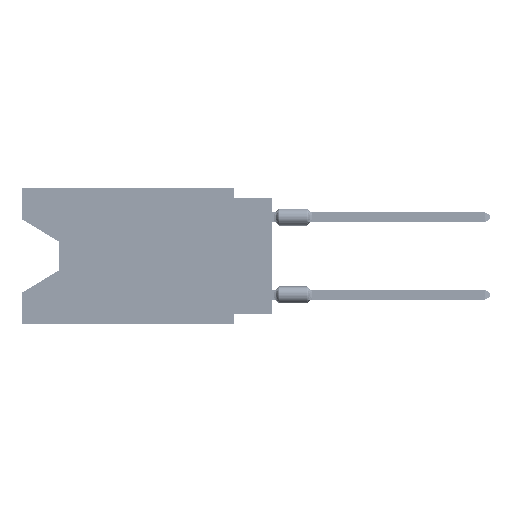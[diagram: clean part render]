
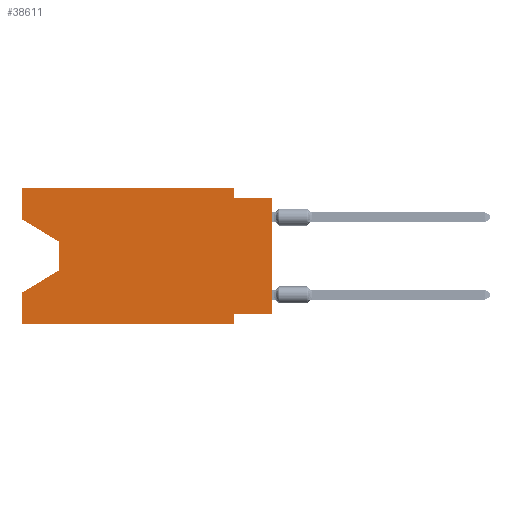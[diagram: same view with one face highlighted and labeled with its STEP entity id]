
A CAD part, left-side view. The second image highlights one B-rep face of the part: STEP entity #38611.
In plain terms, the highlighted planar face has unit normal (-1, 0, 0).
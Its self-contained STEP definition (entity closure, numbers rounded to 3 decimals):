
#2183 = CARTESIAN_POINT ( 'NONE',  ( 0., 2.54, -0.635 ) ) ;
#4354 = EDGE_CURVE ( 'NONE', #25332, #64421, #41586, .T. ) ;
#4647 = EDGE_LOOP ( 'NONE', ( #14590, #85293, #22758, #9300, #32544, #81004, #24702, #36035, #92510, #18713, #27434, #96719 ) ) ;
#5508 = VECTOR ( 'NONE', #71058, 1000. ) ;
#8305 = DIRECTION ( 'NONE',  ( 0., 0., 1. ) ) ;
#8428 = VECTOR ( 'NONE', #8305, 1000. ) ;
#9300 = ORIENTED_EDGE ( 'NONE', *, *, #54876, .F. ) ;
#11261 = EDGE_CURVE ( 'NONE', #54939, #77517, #31250, .T. ) ;
#13982 = CARTESIAN_POINT ( 'NONE',  ( 0., 16.383, -8.89 ) ) ;
#14084 = CARTESIAN_POINT ( 'NONE',  ( 0., 16.383, 0. ) ) ;
#14590 = ORIENTED_EDGE ( 'NONE', *, *, #80963, .T. ) ;
#15507 = LINE ( 'NONE', #75867, #44547 ) ;
#16127 = VECTOR ( 'NONE', #97850, 1000. ) ;
#16807 = VECTOR ( 'NONE', #97459, 1000. ) ;
#16963 = PLANE ( 'NONE',  #18450 ) ;
#18450 = AXIS2_PLACEMENT_3D ( 'NONE', #32440, #55867, #62850 ) ;
#18713 = ORIENTED_EDGE ( 'NONE', *, *, #30971, .F. ) ;
#20438 = CARTESIAN_POINT ( 'NONE',  ( 0., 2.54, 0. ) ) ;
#21786 = EDGE_CURVE ( 'NONE', #24585, #88785, #82406, .T. ) ;
#22758 = ORIENTED_EDGE ( 'NONE', *, *, #77411, .T. ) ;
#24585 = VERTEX_POINT ( 'NONE', #67412 ) ;
#24702 = ORIENTED_EDGE ( 'NONE', *, *, #63121, .F. ) ;
#25153 = CARTESIAN_POINT ( 'NONE',  ( 0., 16.383, -8.89 ) ) ;
#25172 = DIRECTION ( 'NONE',  ( 0., 1., 0. ) ) ;
#25332 = VERTEX_POINT ( 'NONE', #95007 ) ;
#26108 = CARTESIAN_POINT ( 'NONE',  ( 0., 13.97, -3.505 ) ) ;
#27434 = ORIENTED_EDGE ( 'NONE', *, *, #94796, .F. ) ;
#28334 = VECTOR ( 'NONE', #46251, 1000. ) ;
#30971 = EDGE_CURVE ( 'NONE', #33474, #76440, #81770, .T. ) ;
#31250 = LINE ( 'NONE', #76622, #8428 ) ;
#32107 = DIRECTION ( 'NONE',  ( 0., -1., 0. ) ) ;
#32440 = CARTESIAN_POINT ( 'NONE',  ( 0., 16.383, 0. ) ) ;
#32544 = ORIENTED_EDGE ( 'NONE', *, *, #86923, .T. ) ;
#33474 = VERTEX_POINT ( 'NONE', #43548 ) ;
#34459 = VERTEX_POINT ( 'NONE', #25153 ) ;
#35404 = CARTESIAN_POINT ( 'NONE',  ( 0., 16.383, -2.038 ) ) ;
#36035 = ORIENTED_EDGE ( 'NONE', *, *, #11261, .T. ) ;
#36974 = EDGE_CURVE ( 'NONE', #76440, #77517, #76984, .T. ) ;
#37620 = LINE ( 'NONE', #89989, #16807 ) ;
#37853 = VECTOR ( 'NONE', #43571, 1000. ) ;
#38611 = ADVANCED_FACE ( 'NONE', ( #63337 ), #16963, .F. ) ;
#40628 = LINE ( 'NONE', #78994, #85141 ) ;
#41586 = LINE ( 'NONE', #26108, #28334 ) ;
#43147 = VECTOR ( 'NONE', #88784, 1000. ) ;
#43548 = CARTESIAN_POINT ( 'NONE',  ( 0., 2.54, 0. ) ) ;
#43571 = DIRECTION ( 'NONE',  ( 0., 0., 1. ) ) ;
#43998 = DIRECTION ( 'NONE',  ( 0., -1., 0. ) ) ;
#44547 = VECTOR ( 'NONE', #43998, 1000. ) ;
#46251 = DIRECTION ( 'NONE',  ( 0., 0., -1. ) ) ;
#51066 = CARTESIAN_POINT ( 'NONE',  ( 0., 13.97, -5.385 ) ) ;
#52609 = CARTESIAN_POINT ( 'NONE',  ( 0., 0., -0.635 ) ) ;
#54491 = CARTESIAN_POINT ( 'NONE',  ( 0., 16.383, -6.852 ) ) ;
#54876 = EDGE_CURVE ( 'NONE', #34459, #63399, #90419, .T. ) ;
#54939 = VERTEX_POINT ( 'NONE', #93355 ) ;
#55867 = DIRECTION ( 'NONE',  ( 1., 0., 0. ) ) ;
#62258 = VECTOR ( 'NONE', #73878, 1000. ) ;
#62850 = DIRECTION ( 'NONE',  ( 0., 0., -1. ) ) ;
#63121 = EDGE_CURVE ( 'NONE', #54939, #24585, #40628, .T. ) ;
#63337 = FACE_OUTER_BOUND ( 'NONE', #4647, .T. ) ;
#63399 = VERTEX_POINT ( 'NONE', #54491 ) ;
#64421 = VERTEX_POINT ( 'NONE', #51066 ) ;
#65108 = DIRECTION ( 'NONE',  ( 0., 0.855, -0.519 ) ) ;
#65611 = CARTESIAN_POINT ( 'NONE',  ( 0., 13.97, -5.385 ) ) ;
#66101 = LINE ( 'NONE', #65611, #96582 ) ;
#67412 = CARTESIAN_POINT ( 'NONE',  ( 0., 2.54, -8.255 ) ) ;
#68366 = VERTEX_POINT ( 'NONE', #93583 ) ;
#69507 = CARTESIAN_POINT ( 'NONE',  ( 0., 0., -0.635 ) ) ;
#71058 = DIRECTION ( 'NONE',  ( 0., 0., 1. ) ) ;
#73878 = DIRECTION ( 'NONE',  ( 0., -1., 0. ) ) ;
#74101 = CARTESIAN_POINT ( 'NONE',  ( 0., 2.54, -8.89 ) ) ;
#75867 = CARTESIAN_POINT ( 'NONE',  ( 0., 16.383, 0. ) ) ;
#75901 = CARTESIAN_POINT ( 'NONE',  ( 0., 2.54, -8.89 ) ) ;
#76440 = VERTEX_POINT ( 'NONE', #2183 ) ;
#76622 = CARTESIAN_POINT ( 'NONE',  ( 0., 0., 0. ) ) ;
#76984 = LINE ( 'NONE', #69507, #98123 ) ;
#77411 = EDGE_CURVE ( 'NONE', #64421, #63399, #66101, .T. ) ;
#77517 = VERTEX_POINT ( 'NONE', #52609 ) ;
#78539 = CARTESIAN_POINT ( 'NONE',  ( 0., 16.383, 0. ) ) ;
#78994 = CARTESIAN_POINT ( 'NONE',  ( 0., 0., -8.255 ) ) ;
#80963 = EDGE_CURVE ( 'NONE', #83447, #25332, #37620, .T. ) ;
#81004 = ORIENTED_EDGE ( 'NONE', *, *, #21786, .F. ) ;
#81770 = LINE ( 'NONE', #20438, #43147 ) ;
#82406 = LINE ( 'NONE', #75901, #16127 ) ;
#83325 = LINE ( 'NONE', #13982, #62258 ) ;
#83447 = VERTEX_POINT ( 'NONE', #35404 ) ;
#85054 = LINE ( 'NONE', #78539, #5508 ) ;
#85141 = VECTOR ( 'NONE', #25172, 1000. ) ;
#85293 = ORIENTED_EDGE ( 'NONE', *, *, #4354, .T. ) ;
#86923 = EDGE_CURVE ( 'NONE', #34459, #88785, #83325, .T. ) ;
#88784 = DIRECTION ( 'NONE',  ( 0., 0., -1. ) ) ;
#88785 = VERTEX_POINT ( 'NONE', #74101 ) ;
#89989 = CARTESIAN_POINT ( 'NONE',  ( 0., 16.383, -2.038 ) ) ;
#90419 = LINE ( 'NONE', #14084, #37853 ) ;
#92510 = ORIENTED_EDGE ( 'NONE', *, *, #36974, .F. ) ;
#92897 = EDGE_CURVE ( 'NONE', #83447, #68366, #85054, .T. ) ;
#93355 = CARTESIAN_POINT ( 'NONE',  ( 0., 0., -8.255 ) ) ;
#93583 = CARTESIAN_POINT ( 'NONE',  ( 0., 16.383, 0. ) ) ;
#94796 = EDGE_CURVE ( 'NONE', #68366, #33474, #15507, .T. ) ;
#95007 = CARTESIAN_POINT ( 'NONE',  ( 0., 13.97, -3.505 ) ) ;
#96582 = VECTOR ( 'NONE', #65108, 1000. ) ;
#96719 = ORIENTED_EDGE ( 'NONE', *, *, #92897, .F. ) ;
#97459 = DIRECTION ( 'NONE',  ( 0., -0.855, -0.519 ) ) ;
#97850 = DIRECTION ( 'NONE',  ( 0., 0., -1. ) ) ;
#98123 = VECTOR ( 'NONE', #32107, 1000. ) ;
